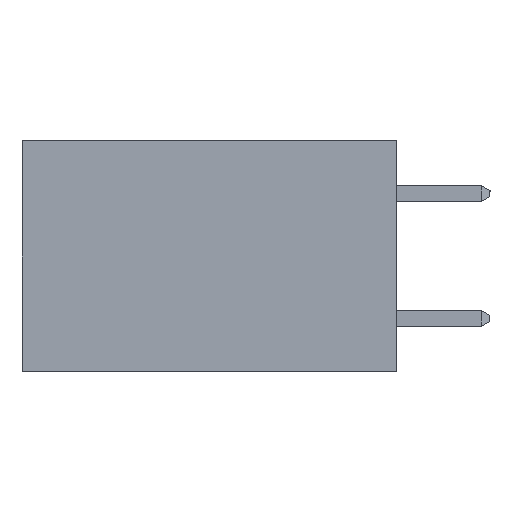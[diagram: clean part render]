
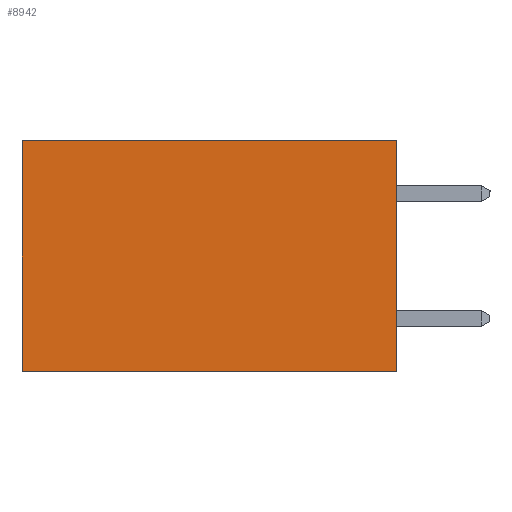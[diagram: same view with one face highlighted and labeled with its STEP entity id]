
A CAD part, left-side view. The second image highlights one B-rep face of the part: STEP entity #8942.
In plain terms, the highlighted planar face has unit normal (-1, 0, 0).
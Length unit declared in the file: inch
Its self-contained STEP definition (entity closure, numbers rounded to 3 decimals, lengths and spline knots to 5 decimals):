
#1860 = LINE ( 'NONE', #3282, #9823 ) ;
#2124 = DIRECTION ( 'NONE',  ( 0., 0., -1. ) ) ;
#2353 = LINE ( 'NONE', #11382, #21483 ) ;
#2397 = VECTOR ( 'NONE', #2124, 39.37008 ) ;
#3282 = CARTESIAN_POINT ( 'NONE',  ( 0.2615, 0.6, -0.37 ) ) ;
#4518 = EDGE_LOOP ( 'NONE', ( #11913, #12192, #12325, #19724 ) ) ;
#4859 = VERTEX_POINT ( 'NONE', #14029 ) ;
#5048 = VERTEX_POINT ( 'NONE', #18137 ) ;
#5321 = LINE ( 'NONE', #14336, #20777 ) ;
#6528 = DIRECTION ( 'NONE',  ( 1., 0., 0. ) ) ;
#7962 = PLANE ( 'NONE',  #12972 ) ;
#8303 = FACE_OUTER_BOUND ( 'NONE', #4518, .T. ) ;
#8389 = EDGE_CURVE ( 'NONE', #9770, #4859, #17741, .T. ) ;
#8435 = EDGE_CURVE ( 'NONE', #4859, #5048, #5321, .T. ) ;
#8942 = ADVANCED_FACE ( 'NONE', ( #8303 ), #7962, .F. ) ;
#9770 = VERTEX_POINT ( 'NONE', #21769 ) ;
#9823 = VECTOR ( 'NONE', #16074, 39.37008 ) ;
#11382 = CARTESIAN_POINT ( 'NONE',  ( 0.2615, 0., 0. ) ) ;
#11876 = CARTESIAN_POINT ( 'NONE',  ( 0.2615, 0., -0.37 ) ) ;
#11913 = ORIENTED_EDGE ( 'NONE', *, *, #21370, .T. ) ;
#12192 = ORIENTED_EDGE ( 'NONE', *, *, #8435, .F. ) ;
#12325 = ORIENTED_EDGE ( 'NONE', *, *, #8389, .F. ) ;
#12459 = DIRECTION ( 'NONE',  ( 0., 1., 0. ) ) ;
#12972 = AXIS2_PLACEMENT_3D ( 'NONE', #22387, #6528, #13221 ) ;
#13221 = DIRECTION ( 'NONE',  ( 0., 0., -1. ) ) ;
#14029 = CARTESIAN_POINT ( 'NONE',  ( 0.2615, 0., -0.37 ) ) ;
#14336 = CARTESIAN_POINT ( 'NONE',  ( 0.2615, 0., -0.37 ) ) ;
#16043 = CARTESIAN_POINT ( 'NONE',  ( 0.2615, 0.6, 0. ) ) ;
#16074 = DIRECTION ( 'NONE',  ( 0., 0., -1. ) ) ;
#17741 = LINE ( 'NONE', #11876, #2397 ) ;
#18137 = CARTESIAN_POINT ( 'NONE',  ( 0.2615, 0.6, -0.37 ) ) ;
#19724 = ORIENTED_EDGE ( 'NONE', *, *, #22710, .T. ) ;
#20415 = VERTEX_POINT ( 'NONE', #16043 ) ;
#20777 = VECTOR ( 'NONE', #12459, 39.37008 ) ;
#21370 = EDGE_CURVE ( 'NONE', #20415, #5048, #1860, .T. ) ;
#21483 = VECTOR ( 'NONE', #22318, 39.37008 ) ;
#21769 = CARTESIAN_POINT ( 'NONE',  ( 0.2615, 0., 0. ) ) ;
#22318 = DIRECTION ( 'NONE',  ( 0., 1., 0. ) ) ;
#22387 = CARTESIAN_POINT ( 'NONE',  ( 0.2615, 0., -0.37 ) ) ;
#22710 = EDGE_CURVE ( 'NONE', #9770, #20415, #2353, .T. ) ;
